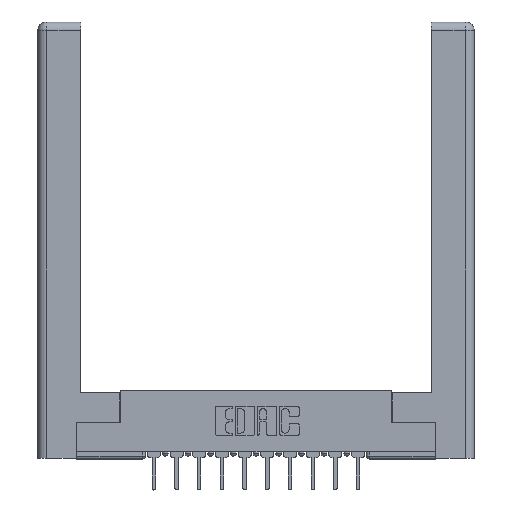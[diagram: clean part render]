
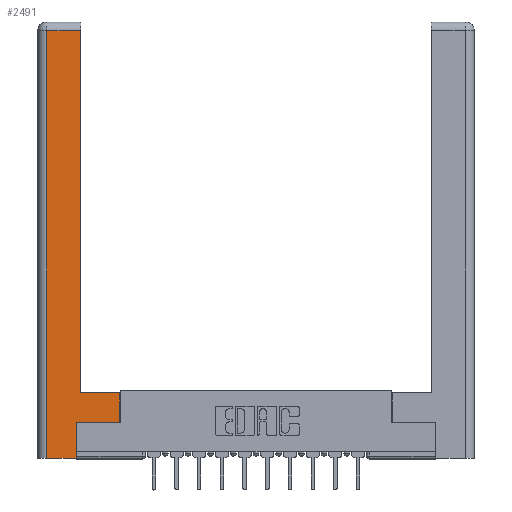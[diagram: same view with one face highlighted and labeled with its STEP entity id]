
A CAD part, top view. The second image highlights one B-rep face of the part: STEP entity #2491.
In plain terms, the highlighted planar face has unit normal (0, 0, 1).
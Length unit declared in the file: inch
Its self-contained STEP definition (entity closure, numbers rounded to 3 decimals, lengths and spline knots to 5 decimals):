
#325 = VECTOR ( 'NONE', #7381, 39.37008 ) ;
#353 = CARTESIAN_POINT ( 'NONE',  ( 0.295, 0.45, 0. ) ) ;
#627 = VECTOR ( 'NONE', #9490, 39.37008 ) ;
#685 = CARTESIAN_POINT ( 'NONE',  ( 0.0615, 0., 0. ) ) ;
#711 = LINE ( 'NONE', #353, #14598 ) ;
#737 = CARTESIAN_POINT ( 'NONE',  ( 0.295, 0.45, 0. ) ) ;
#797 = DIRECTION ( 'NONE',  ( -1., 0., 0. ) ) ;
#893 = AXIS2_PLACEMENT_3D ( 'NONE', #8013, #987, #797 ) ;
#987 = DIRECTION ( 'NONE',  ( 0., 0., -1. ) ) ;
#1089 = ORIENTED_EDGE ( 'NONE', *, *, #2412, .T. ) ;
#1224 = EDGE_CURVE ( 'NONE', #13148, #2054, #13827, .T. ) ;
#1386 = VERTEX_POINT ( 'NONE', #5196 ) ;
#1434 = ORIENTED_EDGE ( 'NONE', *, *, #8377, .T. ) ;
#1487 = CARTESIAN_POINT ( 'NONE',  ( 0.295, 3., 0. ) ) ;
#2046 = DIRECTION ( 'NONE',  ( -1., 0., 0. ) ) ;
#2054 = VERTEX_POINT ( 'NONE', #2766 ) ;
#2217 = EDGE_CURVE ( 'NONE', #4764, #13329, #2249, .T. ) ;
#2249 = LINE ( 'NONE', #14894, #7968 ) ;
#2303 = VERTEX_POINT ( 'NONE', #5673 ) ;
#2412 = EDGE_CURVE ( 'NONE', #1386, #2303, #13409, .T. ) ;
#2491 = ADVANCED_FACE ( 'NONE', ( #7938 ), #6838, .F. ) ;
#2766 = CARTESIAN_POINT ( 'NONE',  ( 0.565, 0.245, 0. ) ) ;
#3284 = CARTESIAN_POINT ( 'NONE',  ( 0.0615, 2.94, 0. ) ) ;
#3725 = CARTESIAN_POINT ( 'NONE',  ( 0.265, 0.245, 0. ) ) ;
#3777 = CARTESIAN_POINT ( 'NONE',  ( 0.565, 0.245, 0. ) ) ;
#3836 = LINE ( 'NONE', #8006, #7342 ) ;
#4256 = CARTESIAN_POINT ( 'NONE',  ( 0.0615, 0., 0. ) ) ;
#4258 = ORIENTED_EDGE ( 'NONE', *, *, #5132, .T. ) ;
#4764 = VERTEX_POINT ( 'NONE', #4256 ) ;
#5004 = VECTOR ( 'NONE', #2046, 39.37008 ) ;
#5132 = EDGE_CURVE ( 'NONE', #12654, #1386, #6870, .T. ) ;
#5164 = DIRECTION ( 'NONE',  ( -1., 0., 0. ) ) ;
#5196 = CARTESIAN_POINT ( 'NONE',  ( 0.295, 2.94, 0. ) ) ;
#5319 = ORIENTED_EDGE ( 'NONE', *, *, #1224, .T. ) ;
#5558 = CARTESIAN_POINT ( 'NONE',  ( 0.265, 0., 0. ) ) ;
#5673 = CARTESIAN_POINT ( 'NONE',  ( 0.0615, 2.94, 0. ) ) ;
#6380 = DIRECTION ( 'NONE',  ( 0., -1., 0. ) ) ;
#6759 = ORIENTED_EDGE ( 'NONE', *, *, #13074, .T. ) ;
#6838 = PLANE ( 'NONE',  #893 ) ;
#6870 = LINE ( 'NONE', #1487, #627 ) ;
#7014 = ORIENTED_EDGE ( 'NONE', *, *, #2217, .T. ) ;
#7342 = VECTOR ( 'NONE', #11380, 39.37008 ) ;
#7381 = DIRECTION ( 'NONE',  ( 0., 1., 0. ) ) ;
#7938 = FACE_OUTER_BOUND ( 'NONE', #14453, .T. ) ;
#7968 = VECTOR ( 'NONE', #13744, 39.37008 ) ;
#8006 = CARTESIAN_POINT ( 'NONE',  ( 0.565, 0.45, 0. ) ) ;
#8013 = CARTESIAN_POINT ( 'NONE',  ( 0., 0., 0. ) ) ;
#8377 = EDGE_CURVE ( 'NONE', #2303, #4764, #10187, .T. ) ;
#8937 = ORIENTED_EDGE ( 'NONE', *, *, #14915, .T. ) ;
#9012 = ORIENTED_EDGE ( 'NONE', *, *, #12744, .T. ) ;
#9490 = DIRECTION ( 'NONE',  ( 0., 1., 0. ) ) ;
#9861 = LINE ( 'NONE', #3725, #325 ) ;
#9882 = CARTESIAN_POINT ( 'NONE',  ( 0.265, 0.245, 0. ) ) ;
#10102 = VERTEX_POINT ( 'NONE', #12862 ) ;
#10187 = LINE ( 'NONE', #685, #14199 ) ;
#10650 = DIRECTION ( 'NONE',  ( 1., 0., 0. ) ) ;
#11380 = DIRECTION ( 'NONE',  ( 0., 1., 0. ) ) ;
#12654 = VERTEX_POINT ( 'NONE', #737 ) ;
#12744 = EDGE_CURVE ( 'NONE', #2054, #10102, #3836, .T. ) ;
#12862 = CARTESIAN_POINT ( 'NONE',  ( 0.565, 0.45, 0. ) ) ;
#13074 = EDGE_CURVE ( 'NONE', #10102, #12654, #711, .T. ) ;
#13148 = VERTEX_POINT ( 'NONE', #9882 ) ;
#13329 = VERTEX_POINT ( 'NONE', #5558 ) ;
#13409 = LINE ( 'NONE', #3284, #5004 ) ;
#13744 = DIRECTION ( 'NONE',  ( 1., 0., 0. ) ) ;
#13827 = LINE ( 'NONE', #3777, #14543 ) ;
#14199 = VECTOR ( 'NONE', #6380, 39.37008 ) ;
#14453 = EDGE_LOOP ( 'NONE', ( #4258, #1089, #1434, #7014, #8937, #5319, #9012, #6759 ) ) ;
#14543 = VECTOR ( 'NONE', #10650, 39.37008 ) ;
#14598 = VECTOR ( 'NONE', #5164, 39.37008 ) ;
#14894 = CARTESIAN_POINT ( 'NONE',  ( 0.265, 0., 0. ) ) ;
#14915 = EDGE_CURVE ( 'NONE', #13329, #13148, #9861, .T. ) ;
